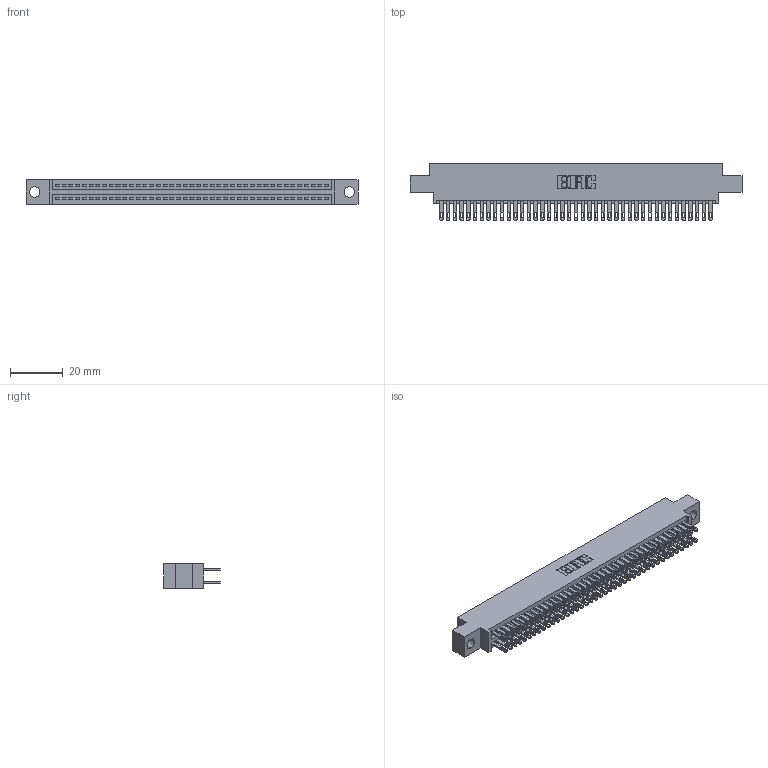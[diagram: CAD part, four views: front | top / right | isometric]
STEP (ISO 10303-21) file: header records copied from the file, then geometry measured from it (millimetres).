
FILE_DESCRIPTION (( 'STEP AP203' ), '1' );
FILE_NAME ('345-082-500-804.STEP', '2021-05-20T11:48:18', ( '' ), ( '' ), 'SwSTEP 2.0', 'SolidWorks 2020', '' );
FILE_SCHEMA (( 'CONFIG_CONTROL_DESIGN' ));
Length unit declared in the file: inch
Products named in the file (3): 345 Part_0.170 Offset - 0.156 Dia-TI; 345-082-500-804; 345-292-001_345-293-100
Assembly tree (83 placements, depth 2):
  345-082-500-804
    345 Part_0.170 Offset - 0.156 Dia-TI
    345-292-001_345-293-100  x82
Bounding box: 125.35 x 21.51 x 9.4 mm (x, y, z)
Volume: 12198.5 mm3; surface area: 18843.5 mm2
Topology: 83 solids, 83 shells, 3916 faces, 11951 edges, 7966 vertices
Faces by surface type: plane 2312, cylinder 1604
Entity records: 32785 total; most frequent: CARTESIAN_POINT 5502, ORIENTED_EDGE 5434, DIRECTION 4853, EDGE_CURVE 2717, LINE 2417, VECTOR 2417, VERTEX_POINT 1810, AXIS2_PLACEMENT_3D 1218
